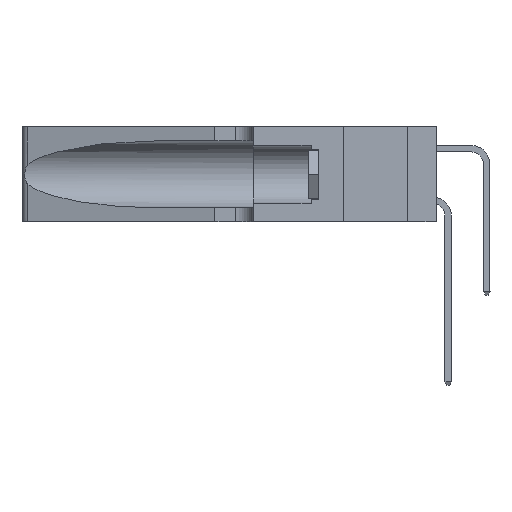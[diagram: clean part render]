
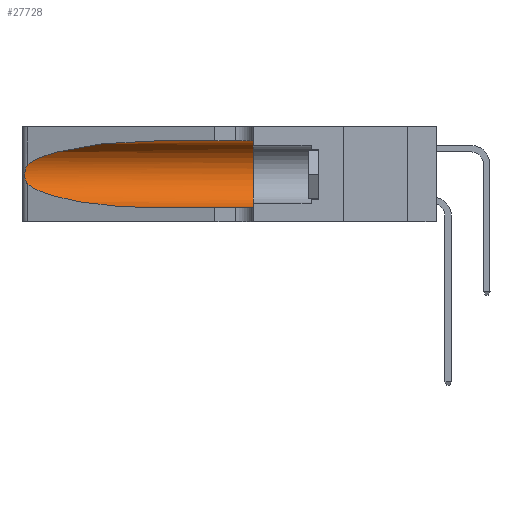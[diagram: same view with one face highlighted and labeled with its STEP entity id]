
A CAD part, left-side view. The second image highlights one B-rep face of the part: STEP entity #27728.
In plain terms, the highlighted cylindrical face has radius 3.308 mm (diameter 6.617 mm), a partial arc.
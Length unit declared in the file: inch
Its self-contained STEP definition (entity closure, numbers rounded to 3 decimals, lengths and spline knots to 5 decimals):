
#424 = ORIENTED_EDGE ( 'NONE', *, *, #34654, .T. ) ;
#1702 = CARTESIAN_POINT ( 'NONE',  ( 0.25787, 1.23484, 0.2124 ) ) ;
#3362 = CARTESIAN_POINT ( 'NONE',  ( 0.25487, 1.22718, 0.22369 ) ) ;
#6238 = CARTESIAN_POINT ( 'NONE',  ( 0.25639, 1.23186, 0.15144 ) ) ;
#7035 = VECTOR ( 'NONE', #13161, 39.37008 ) ;
#7053 = CARTESIAN_POINT ( 'NONE',  ( 0.1305, 0.72297, 0.31525 ) ) ;
#7907 = AXIS2_PLACEMENT_3D ( 'NONE', #38165, #29493, #10322 ) ;
#8547 = CARTESIAN_POINT ( 'NONE',  ( 0.2373, 1.15595, 0.08982 ) ) ;
#8615 = CARTESIAN_POINT ( 'NONE',  ( 0.26075, 1.23896, 0.178 ) ) ;
#8739 =( BOUNDED_CURVE ( )  B_SPLINE_CURVE ( 3, ( #31093, #8547, #18465, #40994 ),
 .UNSPECIFIED., .F., .F. ) 
 B_SPLINE_CURVE_WITH_KNOTS ( ( 4, 4 ),
 ( 3.44316, 4.71239 ),
 .UNSPECIFIED. ) 
 CURVE ( )  GEOMETRIC_REPRESENTATION_ITEM ( )  RATIONAL_B_SPLINE_CURVE ( ( 1., 0.87, 0.87, 1. ) ) 
 REPRESENTATION_ITEM ( '' )  );
#8759 = CARTESIAN_POINT ( 'NONE',  ( 0.26075, 1.23896, 0.19203 ) ) ;
#9635 = VERTEX_POINT ( 'NONE', #34350 ) ;
#9856 = VERTEX_POINT ( 'NONE', #3362 ) ;
#10322 = DIRECTION ( 'NONE',  ( 0., 0., 1. ) ) ;
#10943 = CARTESIAN_POINT ( 'NONE',  ( 0.18966, 0.96281, 0.31525 ) ) ;
#11230 = CARTESIAN_POINT ( 'NONE',  ( 0.1305, 0.72297, 0.31525 ) ) ;
#11800 = CARTESIAN_POINT ( 'NONE',  ( 0.1305, 0.72297, 0.05475 ) ) ;
#12010 = DIRECTION ( 'NONE',  ( 0., 0., -1. ) ) ;
#12317 = VERTEX_POINT ( 'NONE', #7053 ) ;
#12502 = CARTESIAN_POINT ( 'NONE',  ( 0.25487, 1.22718, 0.14631 ) ) ;
#13020 = FACE_OUTER_BOUND ( 'NONE', #14081, .T. ) ;
#13161 = DIRECTION ( 'NONE',  ( 0., -1., 0. ) ) ;
#13246 = AXIS2_PLACEMENT_3D ( 'NONE', #14101, #17294, #12010 ) ;
#13946 = VERTEX_POINT ( 'NONE', #30935 ) ;
#14029 = EDGE_CURVE ( 'NONE', #9856, #13946, #16643, .T. ) ;
#14081 = EDGE_LOOP ( 'NONE', ( #27305, #19464, #18412, #424, #35368, #30300 ) ) ;
#14101 = CARTESIAN_POINT ( 'NONE',  ( 0.1305, 1.61858, 0.185 ) ) ;
#14210 = CARTESIAN_POINT ( 'NONE',  ( 0.25639, 1.23184, 0.21858 ) ) ;
#14576 = CARTESIAN_POINT ( 'NONE',  ( 0.1305, 1.61858, 0.31525 ) ) ;
#15043 = CARTESIAN_POINT ( 'NONE',  ( 0.25856, 1.23593, 0.16098 ) ) ;
#15051 = CYLINDRICAL_SURFACE ( 'NONE', #13246, 0.13025 ) ;
#15567 = LINE ( 'NONE', #28906, #7035 ) ;
#16392 = CIRCLE ( 'NONE', #7907, 0.13025 ) ;
#16638 = VERTEX_POINT ( 'NONE', #11800 ) ;
#16643 = B_SPLINE_CURVE_WITH_KNOTS ( 'NONE', 3,
 ( #39339, #26262, #14210, #1702, #36689, #24608, #8759, #8615, #31011, #15043, #34486, #6238, #22018, #12502 ),
 .UNSPECIFIED., .F., .F.,
 ( 4, 2, 2, 2, 2, 2, 4 ),
 ( 0., 0.00027, 0.00053, 0.00107, 0.0016, 0.00187, 0.00214 ),
 .UNSPECIFIED. ) ;
#17294 = DIRECTION ( 'NONE',  ( 0., -1., 0. ) ) ;
#17351 = CARTESIAN_POINT ( 'NONE',  ( 0.25487, 1.22718, 0.22369 ) ) ;
#18201 = CARTESIAN_POINT ( 'NONE',  ( 0.1305, 0.35, 0.05475 ) ) ;
#18324 = VECTOR ( 'NONE', #40473, 39.37008 ) ;
#18412 = ORIENTED_EDGE ( 'NONE', *, *, #35086, .T. ) ;
#18465 = CARTESIAN_POINT ( 'NONE',  ( 0.18966, 0.96281, 0.05475 ) ) ;
#19464 = ORIENTED_EDGE ( 'NONE', *, *, #14029, .T. ) ;
#22018 = CARTESIAN_POINT ( 'NONE',  ( 0.25555, 1.22993, 0.14849 ) ) ;
#24189 = EDGE_CURVE ( 'NONE', #12317, #9635, #26853, .T. ) ;
#24608 = CARTESIAN_POINT ( 'NONE',  ( 0.26018, 1.23835, 0.19895 ) ) ;
#25227 = EDGE_CURVE ( 'NONE', #12317, #9856, #25444, .T. ) ;
#25444 =( BOUNDED_CURVE ( )  B_SPLINE_CURVE ( 3, ( #11230, #10943, #36492, #17351 ),
 .UNSPECIFIED., .F., .T. ) 
 B_SPLINE_CURVE_WITH_KNOTS ( ( 4, 4 ),
 ( 1.5708, 2.84003 ),
 .UNSPECIFIED. ) 
 CURVE ( )  GEOMETRIC_REPRESENTATION_ITEM ( )  RATIONAL_B_SPLINE_CURVE ( ( 1., 0.87, 0.87, 1. ) ) 
 REPRESENTATION_ITEM ( '' )  );
#26262 = CARTESIAN_POINT ( 'NONE',  ( 0.25555, 1.22994, 0.2215 ) ) ;
#26853 = LINE ( 'NONE', #14576, #18324 ) ;
#27305 = ORIENTED_EDGE ( 'NONE', *, *, #25227, .T. ) ;
#27728 = ADVANCED_FACE ( 'NONE', ( #13020 ), #15051, .F. ) ;
#28906 = CARTESIAN_POINT ( 'NONE',  ( 0.1305, 1.61858, 0.05475 ) ) ;
#29493 = DIRECTION ( 'NONE',  ( 0., 1., 0. ) ) ;
#30101 = VERTEX_POINT ( 'NONE', #18201 ) ;
#30300 = ORIENTED_EDGE ( 'NONE', *, *, #24189, .F. ) ;
#30935 = CARTESIAN_POINT ( 'NONE',  ( 0.25487, 1.22718, 0.14631 ) ) ;
#31011 = CARTESIAN_POINT ( 'NONE',  ( 0.26017, 1.23833, 0.17102 ) ) ;
#31093 = CARTESIAN_POINT ( 'NONE',  ( 0.25487, 1.22718, 0.14631 ) ) ;
#34350 = CARTESIAN_POINT ( 'NONE',  ( 0.1305, 0.35, 0.31525 ) ) ;
#34486 = CARTESIAN_POINT ( 'NONE',  ( 0.25789, 1.23486, 0.15765 ) ) ;
#34654 = EDGE_CURVE ( 'NONE', #16638, #30101, #15567, .T. ) ;
#35086 = EDGE_CURVE ( 'NONE', #13946, #16638, #8739, .T. ) ;
#35368 = ORIENTED_EDGE ( 'NONE', *, *, #36817, .F. ) ;
#36492 = CARTESIAN_POINT ( 'NONE',  ( 0.2373, 1.15595, 0.28018 ) ) ;
#36689 = CARTESIAN_POINT ( 'NONE',  ( 0.25854, 1.2359, 0.20912 ) ) ;
#36817 = EDGE_CURVE ( 'NONE', #9635, #30101, #16392, .T. ) ;
#38165 = CARTESIAN_POINT ( 'NONE',  ( 0.1305, 0.35, 0.185 ) ) ;
#39339 = CARTESIAN_POINT ( 'NONE',  ( 0.25487, 1.22718, 0.22369 ) ) ;
#40473 = DIRECTION ( 'NONE',  ( 0., -1., 0. ) ) ;
#40994 = CARTESIAN_POINT ( 'NONE',  ( 0.1305, 0.72297, 0.05475 ) ) ;
